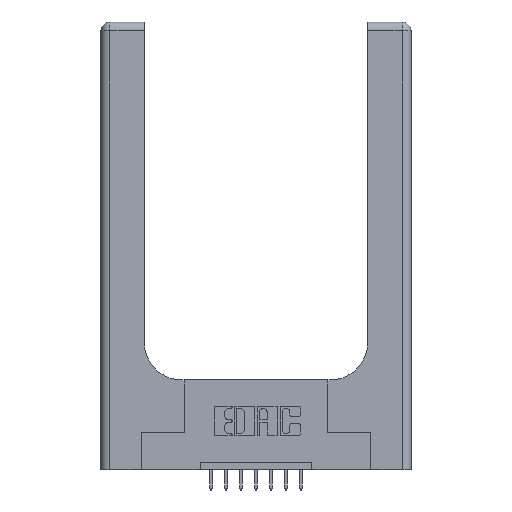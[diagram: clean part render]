
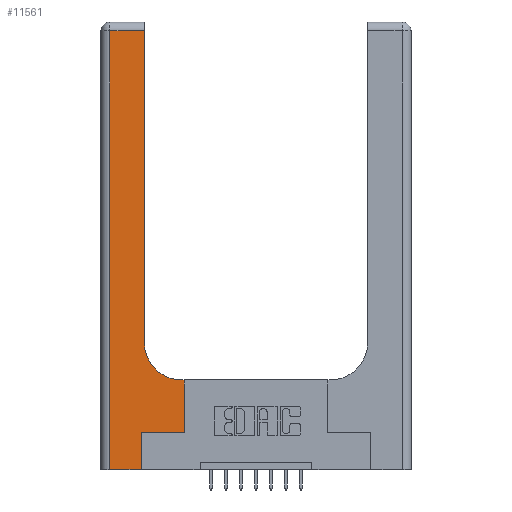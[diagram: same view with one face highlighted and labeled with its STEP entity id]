
A CAD part, top view. The second image highlights one B-rep face of the part: STEP entity #11561.
In plain terms, the highlighted planar face has unit normal (0, 0, 1).
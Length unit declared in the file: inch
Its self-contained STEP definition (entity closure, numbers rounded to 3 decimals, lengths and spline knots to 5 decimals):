
#305 = EDGE_CURVE ( 'NONE', #13676, #10025, #10265, .T. ) ;
#376 = DIRECTION ( 'NONE',  ( -1., 0., 0. ) ) ;
#501 = ORIENTED_EDGE ( 'NONE', *, *, #14429, .T. ) ;
#725 = ORIENTED_EDGE ( 'NONE', *, *, #6459, .T. ) ;
#890 = DIRECTION ( 'NONE',  ( 1., 0., 0. ) ) ;
#1412 = EDGE_CURVE ( 'NONE', #2338, #13676, #8554, .T. ) ;
#1456 = PLANE ( 'NONE',  #6732 ) ;
#1660 = LINE ( 'NONE', #6447, #8127 ) ;
#1742 = LINE ( 'NONE', #7692, #6603 ) ;
#1745 = LINE ( 'NONE', #2684, #6804 ) ;
#1938 = VERTEX_POINT ( 'NONE', #7850 ) ;
#2338 = VERTEX_POINT ( 'NONE', #4337 ) ;
#2609 = CARTESIAN_POINT ( 'NONE',  ( 0.269, 0.25, 0.37 ) ) ;
#2614 = ORIENTED_EDGE ( 'NONE', *, *, #3729, .T. ) ;
#2684 = CARTESIAN_POINT ( 'NONE',  ( 0.269, 0., 0.37 ) ) ;
#3055 = DIRECTION ( 'NONE',  ( -1., 0., 0. ) ) ;
#3138 = CARTESIAN_POINT ( 'NONE',  ( 0.269, 0.25, 0.37 ) ) ;
#3261 = VERTEX_POINT ( 'NONE', #7933 ) ;
#3557 = ORIENTED_EDGE ( 'NONE', *, *, #13323, .T. ) ;
#3729 = EDGE_CURVE ( 'NONE', #10025, #10329, #1742, .T. ) ;
#3843 = VECTOR ( 'NONE', #12737, 39.37008 ) ;
#3958 = CARTESIAN_POINT ( 'NONE',  ( 0.06, 3., 0.37 ) ) ;
#4337 = CARTESIAN_POINT ( 'NONE',  ( 0.5415, 0.6, 0.37 ) ) ;
#4429 = VECTOR ( 'NONE', #890, 39.37008 ) ;
#5019 = DIRECTION ( 'NONE',  ( 1., 0., 0. ) ) ;
#5081 = ORIENTED_EDGE ( 'NONE', *, *, #305, .T. ) ;
#5124 = CARTESIAN_POINT ( 'NONE',  ( 0.2915, 0.85, 0.37 ) ) ;
#5273 = DIRECTION ( 'NONE',  ( 0., -1., 0. ) ) ;
#5712 = VECTOR ( 'NONE', #10144, 39.37008 ) ;
#6447 = CARTESIAN_POINT ( 'NONE',  ( 0.5585, 0.25, 0.37 ) ) ;
#6459 = EDGE_CURVE ( 'NONE', #8191, #1938, #1660, .T. ) ;
#6472 = DIRECTION ( 'NONE',  ( 0., 0., -1. ) ) ;
#6603 = VECTOR ( 'NONE', #3055, 39.37008 ) ;
#6631 = EDGE_CURVE ( 'NONE', #3261, #7101, #13636, .T. ) ;
#6732 = AXIS2_PLACEMENT_3D ( 'NONE', #12030, #6472, #376 ) ;
#6804 = VECTOR ( 'NONE', #9762, 39.37008 ) ;
#7101 = VERTEX_POINT ( 'NONE', #13697 ) ;
#7326 = FACE_OUTER_BOUND ( 'NONE', #12918, .T. ) ;
#7682 = LINE ( 'NONE', #7749, #5712 ) ;
#7692 = CARTESIAN_POINT ( 'NONE',  ( 0., 2.94, 0.37 ) ) ;
#7749 = CARTESIAN_POINT ( 'NONE',  ( 0.2915, 0.6, 0.37 ) ) ;
#7850 = CARTESIAN_POINT ( 'NONE',  ( 0.5585, 0.6, 0.37 ) ) ;
#7922 = CARTESIAN_POINT ( 'NONE',  ( 0.06, 2.94, 0.37 ) ) ;
#7933 = CARTESIAN_POINT ( 'NONE',  ( 0.06, 0., 0.37 ) ) ;
#7987 = CARTESIAN_POINT ( 'NONE',  ( 0.5585, 0.25, 0.37 ) ) ;
#8053 = AXIS2_PLACEMENT_3D ( 'NONE', #9716, #9569, #5019 ) ;
#8127 = VECTOR ( 'NONE', #14417, 39.37008 ) ;
#8191 = VERTEX_POINT ( 'NONE', #7987 ) ;
#8377 = EDGE_CURVE ( 'NONE', #10329, #3261, #14553, .T. ) ;
#8554 = CIRCLE ( 'NONE', #8053, 0.25 ) ;
#8982 = VERTEX_POINT ( 'NONE', #2609 ) ;
#8987 = CARTESIAN_POINT ( 'NONE',  ( 0., 0., 0.37 ) ) ;
#8997 = DIRECTION ( 'NONE',  ( 1., 0., 0. ) ) ;
#9255 = VECTOR ( 'NONE', #8997, 39.37008 ) ;
#9569 = DIRECTION ( 'NONE',  ( 0., 0., -1. ) ) ;
#9706 = ORIENTED_EDGE ( 'NONE', *, *, #8377, .T. ) ;
#9716 = CARTESIAN_POINT ( 'NONE',  ( 0.5415, 0.85, 0.37 ) ) ;
#9762 = DIRECTION ( 'NONE',  ( 0., 1., 0. ) ) ;
#10025 = VERTEX_POINT ( 'NONE', #13769 ) ;
#10111 = ORIENTED_EDGE ( 'NONE', *, *, #10679, .T. ) ;
#10116 = VECTOR ( 'NONE', #5273, 39.37008 ) ;
#10144 = DIRECTION ( 'NONE',  ( -1., 0., 0. ) ) ;
#10265 = LINE ( 'NONE', #11419, #3843 ) ;
#10329 = VERTEX_POINT ( 'NONE', #7922 ) ;
#10649 = ORIENTED_EDGE ( 'NONE', *, *, #1412, .T. ) ;
#10679 = EDGE_CURVE ( 'NONE', #1938, #2338, #7682, .T. ) ;
#11154 = LINE ( 'NONE', #3138, #9255 ) ;
#11419 = CARTESIAN_POINT ( 'NONE',  ( 0.2915, 3., 0.37 ) ) ;
#11561 = ADVANCED_FACE ( 'NONE', ( #7326 ), #1456, .F. ) ;
#12030 = CARTESIAN_POINT ( 'NONE',  ( 0., 3., 0.37 ) ) ;
#12737 = DIRECTION ( 'NONE',  ( 0., 1., 0. ) ) ;
#12918 = EDGE_LOOP ( 'NONE', ( #5081, #2614, #9706, #14184, #3557, #501, #725, #10111, #10649 ) ) ;
#13323 = EDGE_CURVE ( 'NONE', #7101, #8982, #1745, .T. ) ;
#13636 = LINE ( 'NONE', #8987, #4429 ) ;
#13676 = VERTEX_POINT ( 'NONE', #5124 ) ;
#13697 = CARTESIAN_POINT ( 'NONE',  ( 0.269, 0., 0.37 ) ) ;
#13769 = CARTESIAN_POINT ( 'NONE',  ( 0.2915, 2.94, 0.37 ) ) ;
#14184 = ORIENTED_EDGE ( 'NONE', *, *, #6631, .T. ) ;
#14417 = DIRECTION ( 'NONE',  ( 0., 1., 0. ) ) ;
#14429 = EDGE_CURVE ( 'NONE', #8982, #8191, #11154, .T. ) ;
#14553 = LINE ( 'NONE', #3958, #10116 ) ;
